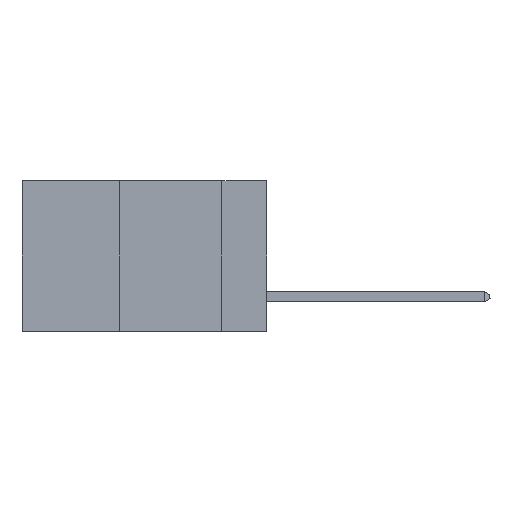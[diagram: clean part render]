
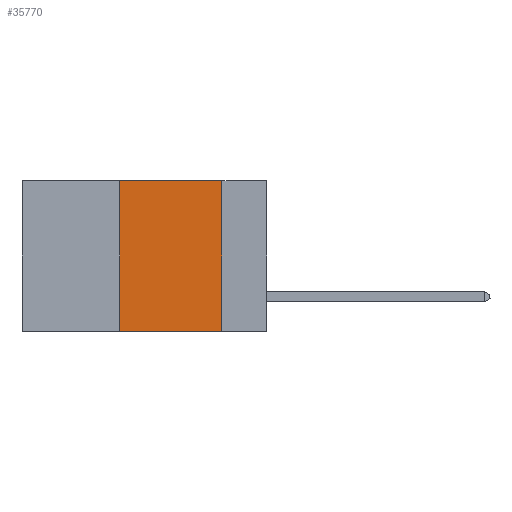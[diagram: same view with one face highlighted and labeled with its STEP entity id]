
A CAD part, left-side view. The second image highlights one B-rep face of the part: STEP entity #35770.
In plain terms, the highlighted planar face has unit normal (-1, 0, 0).
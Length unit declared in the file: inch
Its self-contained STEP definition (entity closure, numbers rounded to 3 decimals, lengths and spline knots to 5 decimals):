
#387 = CARTESIAN_POINT ( 'NONE',  ( 0., 0.36, 0. ) ) ;
#589 = LINE ( 'NONE', #19673, #12709 ) ;
#1304 = VECTOR ( 'NONE', #25029, 39.37008 ) ;
#3636 = CARTESIAN_POINT ( 'NONE',  ( 0., 0.6, 0. ) ) ;
#3929 = VERTEX_POINT ( 'NONE', #33731 ) ;
#4711 = EDGE_CURVE ( 'NONE', #3929, #33962, #28066, .T. ) ;
#5868 = CARTESIAN_POINT ( 'NONE',  ( 0., 0.11, 0. ) ) ;
#6954 = DIRECTION ( 'NONE',  ( 0., 0., -1. ) ) ;
#9794 = EDGE_CURVE ( 'NONE', #34033, #17860, #19554, .T. ) ;
#11060 = FACE_OUTER_BOUND ( 'NONE', #28156, .T. ) ;
#11643 = CARTESIAN_POINT ( 'NONE',  ( 0., 0.36, 0. ) ) ;
#12709 = VECTOR ( 'NONE', #19550, 39.37008 ) ;
#14122 = ORIENTED_EDGE ( 'NONE', *, *, #9794, .F. ) ;
#17246 = CARTESIAN_POINT ( 'NONE',  ( 0., 0.6, -0.37 ) ) ;
#17860 = VERTEX_POINT ( 'NONE', #36409 ) ;
#19251 = VECTOR ( 'NONE', #41348, 39.37008 ) ;
#19550 = DIRECTION ( 'NONE',  ( 0., -1., 0. ) ) ;
#19554 = LINE ( 'NONE', #5868, #37441 ) ;
#19673 = CARTESIAN_POINT ( 'NONE',  ( 0., 0.6, 0. ) ) ;
#20847 = AXIS2_PLACEMENT_3D ( 'NONE', #3636, #33453, #6954 ) ;
#20886 = CARTESIAN_POINT ( 'NONE',  ( 0., 0.11, 0. ) ) ;
#23673 = PLANE ( 'NONE',  #20847 ) ;
#25029 = DIRECTION ( 'NONE',  ( 0., 0., 1. ) ) ;
#25579 = ORIENTED_EDGE ( 'NONE', *, *, #36380, .F. ) ;
#27314 = ORIENTED_EDGE ( 'NONE', *, *, #4711, .F. ) ;
#28066 = LINE ( 'NONE', #11643, #1304 ) ;
#28156 = EDGE_LOOP ( 'NONE', ( #14122, #25579, #27314, #32677 ) ) ;
#29341 = DIRECTION ( 'NONE',  ( 0., 0., -1. ) ) ;
#29613 = EDGE_CURVE ( 'NONE', #3929, #17860, #39780, .T. ) ;
#32677 = ORIENTED_EDGE ( 'NONE', *, *, #29613, .T. ) ;
#33453 = DIRECTION ( 'NONE',  ( 1., 0., 0. ) ) ;
#33731 = CARTESIAN_POINT ( 'NONE',  ( 0., 0.36, -0.37 ) ) ;
#33962 = VERTEX_POINT ( 'NONE', #387 ) ;
#34033 = VERTEX_POINT ( 'NONE', #20886 ) ;
#35770 = ADVANCED_FACE ( 'NONE', ( #11060 ), #23673, .F. ) ;
#36380 = EDGE_CURVE ( 'NONE', #33962, #34033, #589, .T. ) ;
#36409 = CARTESIAN_POINT ( 'NONE',  ( 0., 0.11, -0.37 ) ) ;
#37441 = VECTOR ( 'NONE', #29341, 39.37008 ) ;
#39780 = LINE ( 'NONE', #17246, #19251 ) ;
#41348 = DIRECTION ( 'NONE',  ( 0., -1., 0. ) ) ;
